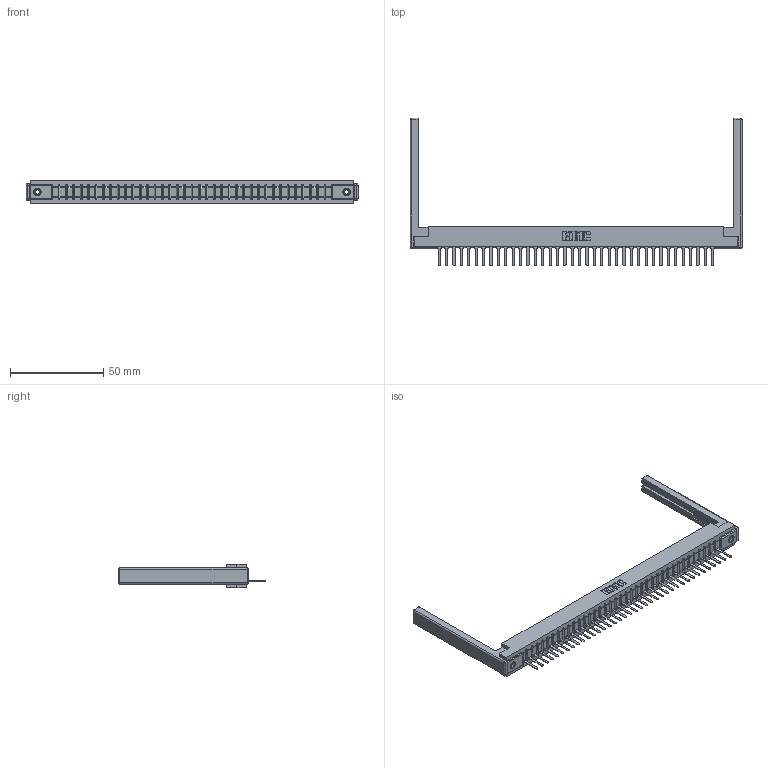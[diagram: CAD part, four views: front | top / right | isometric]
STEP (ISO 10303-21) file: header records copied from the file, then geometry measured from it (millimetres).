
FILE_DESCRIPTION (( 'STEP AP203' ), '1' );
FILE_NAME ('357-038-427-168.STEP', '2020-10-02T20:26:54', ( '' ), ( '' ), 'SwSTEP 2.0', 'SolidWorks 2020', '' );
FILE_SCHEMA (( 'CONFIG_CONTROL_DESIGN' ));
Length unit declared in the file: inch
Products named in the file (5): 307-220-068; 307 Part_.156 Dia Mounting Holes; 345-250-001_345-250-001-102; 307-290-001_527; 357-038-427-168
Assembly tree (43 placements, depth 2):
  357-038-427-168
    307 Part_.156 Dia Mounting Holes
    307-290-001_527  x38
    307-220-068  x2
    345-250-001_345-250-001-102  x2
Bounding box: 178 x 79.07 x 12.7 mm (x, y, z)
Volume: 22872.4 mm3; surface area: 23722.8 mm2
Topology: 43 solids, 43 shells, 2439 faces, 6869 edges, 4402 vertices
Faces by surface type: plane 1564, cylinder 773, sphere 86, cone 12, torus 4
Entity records: 35797 total; most frequent: CARTESIAN_POINT 5993, ORIENTED_EDGE 5968, DIRECTION 5848, EDGE_CURVE 2984, VECTOR 2286, LINE 2286, VERTEX_POINT 1926, AXIS2_PLACEMENT_3D 1781
